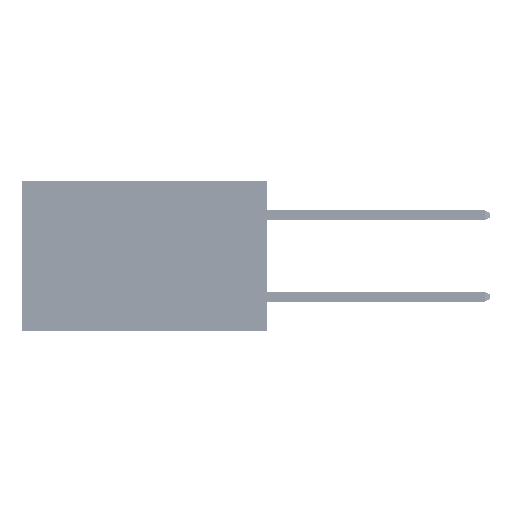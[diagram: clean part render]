
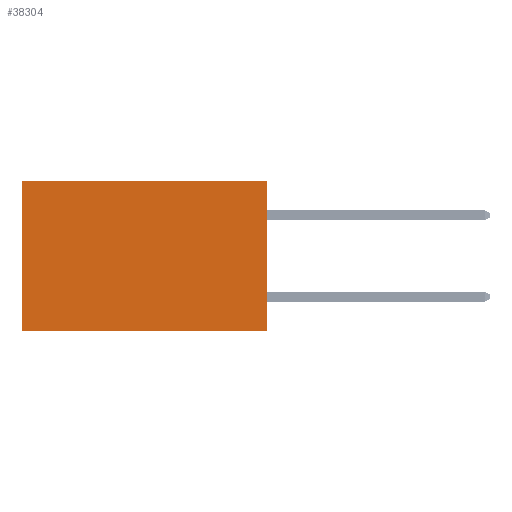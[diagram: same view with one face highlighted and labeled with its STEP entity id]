
A CAD part, left-side view. The second image highlights one B-rep face of the part: STEP entity #38304.
In plain terms, the highlighted planar face has unit normal (-1, 0, 0).
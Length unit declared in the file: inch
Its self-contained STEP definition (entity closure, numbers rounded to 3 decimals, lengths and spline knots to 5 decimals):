
#3325 = EDGE_CURVE ( 'NONE', #50136, #29383, #36563, .T. ) ;
#4946 = LINE ( 'NONE', #14355, #33608 ) ;
#5385 = VERTEX_POINT ( 'NONE', #23008 ) ;
#7273 = PLANE ( 'NONE',  #33216 ) ;
#9229 = CARTESIAN_POINT ( 'NONE',  ( 0.2875, 0.6, 0. ) ) ;
#9610 = ORIENTED_EDGE ( 'NONE', *, *, #22792, .T. ) ;
#12646 = DIRECTION ( 'NONE',  ( 0., 1., 0. ) ) ;
#13235 = LINE ( 'NONE', #9229, #42995 ) ;
#14355 = CARTESIAN_POINT ( 'NONE',  ( 0.2875, 0., 0. ) ) ;
#14831 = CARTESIAN_POINT ( 'NONE',  ( 0.2875, 0., -0.37 ) ) ;
#14911 = LINE ( 'NONE', #15256, #34427 ) ;
#15108 = CARTESIAN_POINT ( 'NONE',  ( 0.2875, 0., 0. ) ) ;
#15256 = CARTESIAN_POINT ( 'NONE',  ( 0.2875, 0., 0. ) ) ;
#16224 = FACE_OUTER_BOUND ( 'NONE', #28743, .T. ) ;
#19041 = DIRECTION ( 'NONE',  ( 0., 0., -1. ) ) ;
#19177 = DIRECTION ( 'NONE',  ( 0., 0., -1. ) ) ;
#22792 = EDGE_CURVE ( 'NONE', #5385, #24662, #4946, .T. ) ;
#23008 = CARTESIAN_POINT ( 'NONE',  ( 0.2875, 0., 0. ) ) ;
#24662 = VERTEX_POINT ( 'NONE', #37486 ) ;
#28743 = EDGE_LOOP ( 'NONE', ( #47855, #29097, #41045, #9610 ) ) ;
#29097 = ORIENTED_EDGE ( 'NONE', *, *, #3325, .F. ) ;
#29383 = VERTEX_POINT ( 'NONE', #38492 ) ;
#32596 = DIRECTION ( 'NONE',  ( 0., 0., -1. ) ) ;
#32614 = EDGE_CURVE ( 'NONE', #5385, #50136, #14911, .T. ) ;
#33216 = AXIS2_PLACEMENT_3D ( 'NONE', #15108, #42235, #19041 ) ;
#33608 = VECTOR ( 'NONE', #49281, 39.37008 ) ;
#34427 = VECTOR ( 'NONE', #19177, 39.37008 ) ;
#35370 = VECTOR ( 'NONE', #12646, 39.37008 ) ;
#36563 = LINE ( 'NONE', #39444, #35370 ) ;
#37486 = CARTESIAN_POINT ( 'NONE',  ( 0.2875, 0.6, 0. ) ) ;
#37748 = EDGE_CURVE ( 'NONE', #24662, #29383, #13235, .T. ) ;
#38304 = ADVANCED_FACE ( 'NONE', ( #16224 ), #7273, .F. ) ;
#38492 = CARTESIAN_POINT ( 'NONE',  ( 0.2875, 0.6, -0.37 ) ) ;
#39444 = CARTESIAN_POINT ( 'NONE',  ( 0.2875, 0., -0.37 ) ) ;
#41045 = ORIENTED_EDGE ( 'NONE', *, *, #32614, .F. ) ;
#42235 = DIRECTION ( 'NONE',  ( 1., 0., 0. ) ) ;
#42995 = VECTOR ( 'NONE', #32596, 39.37008 ) ;
#47855 = ORIENTED_EDGE ( 'NONE', *, *, #37748, .T. ) ;
#49281 = DIRECTION ( 'NONE',  ( 0., 1., 0. ) ) ;
#50136 = VERTEX_POINT ( 'NONE', #14831 ) ;
